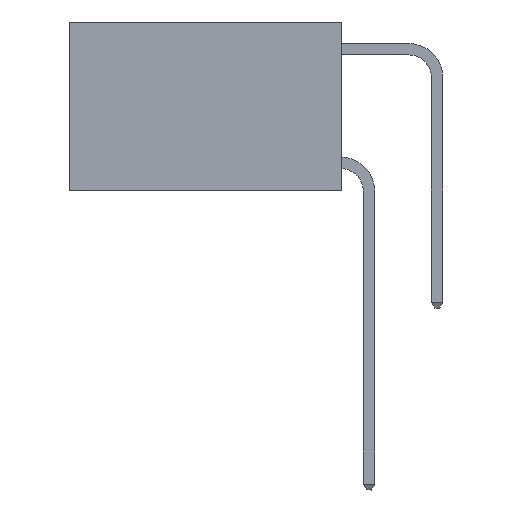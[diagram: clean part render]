
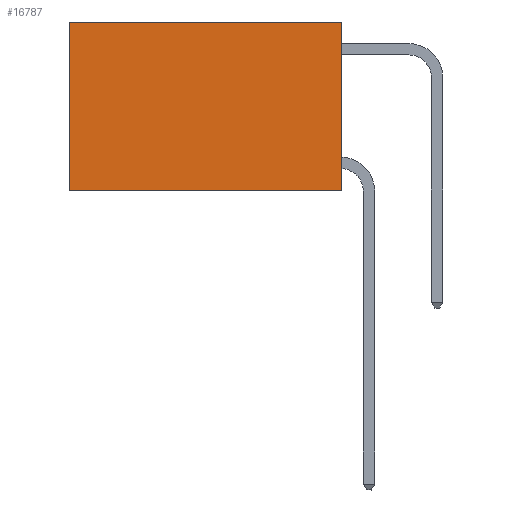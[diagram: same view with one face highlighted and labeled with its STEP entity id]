
A CAD part, left-side view. The second image highlights one B-rep face of the part: STEP entity #16787.
In plain terms, the highlighted planar face has unit normal (-1, 0, 0).
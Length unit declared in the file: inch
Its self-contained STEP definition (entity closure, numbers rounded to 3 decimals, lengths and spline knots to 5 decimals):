
#293 = CARTESIAN_POINT ( 'NONE',  ( 0.2625, 0., 0. ) ) ;
#444 = EDGE_CURVE ( 'NONE', #14229, #8735, #2460, .T. ) ;
#824 = CARTESIAN_POINT ( 'NONE',  ( 0.2625, 0., -0.37 ) ) ;
#1929 = CARTESIAN_POINT ( 'NONE',  ( 0.2625, 0., 0. ) ) ;
#2085 = EDGE_LOOP ( 'NONE', ( #18646, #18537, #19407, #20185 ) ) ;
#2142 = DIRECTION ( 'NONE',  ( 0., 0., -1. ) ) ;
#2460 = LINE ( 'NONE', #824, #11016 ) ;
#3606 = CARTESIAN_POINT ( 'NONE',  ( 0.2625, 0., 0. ) ) ;
#3950 = CARTESIAN_POINT ( 'NONE',  ( 0.2625, 0.6, 0. ) ) ;
#4005 = FACE_OUTER_BOUND ( 'NONE', #2085, .T. ) ;
#6518 = DIRECTION ( 'NONE',  ( 0., 0., -1. ) ) ;
#8426 = DIRECTION ( 'NONE',  ( 0., 1., 0. ) ) ;
#8735 = VERTEX_POINT ( 'NONE', #14678 ) ;
#8857 = EDGE_CURVE ( 'NONE', #22630, #14229, #11913, .T. ) ;
#9423 = DIRECTION ( 'NONE',  ( 0., 0., -1. ) ) ;
#9648 = VECTOR ( 'NONE', #6518, 39.37008 ) ;
#11016 = VECTOR ( 'NONE', #8426, 39.37008 ) ;
#11290 = AXIS2_PLACEMENT_3D ( 'NONE', #12656, #20361, #9423 ) ;
#11356 = VECTOR ( 'NONE', #2142, 39.37008 ) ;
#11913 = LINE ( 'NONE', #293, #11356 ) ;
#12656 = CARTESIAN_POINT ( 'NONE',  ( 0.2625, 0., 0. ) ) ;
#13918 = LINE ( 'NONE', #15612, #9648 ) ;
#14229 = VERTEX_POINT ( 'NONE', #16975 ) ;
#14528 = DIRECTION ( 'NONE',  ( 0., 1., 0. ) ) ;
#14678 = CARTESIAN_POINT ( 'NONE',  ( 0.2625, 0.6, -0.37 ) ) ;
#15612 = CARTESIAN_POINT ( 'NONE',  ( 0.2625, 0.6, 0. ) ) ;
#15707 = LINE ( 'NONE', #3606, #20563 ) ;
#16787 = ADVANCED_FACE ( 'NONE', ( #4005 ), #18216, .F. ) ;
#16975 = CARTESIAN_POINT ( 'NONE',  ( 0.2625, 0., -0.37 ) ) ;
#17814 = EDGE_CURVE ( 'NONE', #21885, #8735, #13918, .T. ) ;
#18216 = PLANE ( 'NONE',  #11290 ) ;
#18537 = ORIENTED_EDGE ( 'NONE', *, *, #444, .F. ) ;
#18646 = ORIENTED_EDGE ( 'NONE', *, *, #17814, .T. ) ;
#19407 = ORIENTED_EDGE ( 'NONE', *, *, #8857, .F. ) ;
#20185 = ORIENTED_EDGE ( 'NONE', *, *, #20463, .T. ) ;
#20361 = DIRECTION ( 'NONE',  ( 1., 0., 0. ) ) ;
#20463 = EDGE_CURVE ( 'NONE', #22630, #21885, #15707, .T. ) ;
#20563 = VECTOR ( 'NONE', #14528, 39.37008 ) ;
#21885 = VERTEX_POINT ( 'NONE', #3950 ) ;
#22630 = VERTEX_POINT ( 'NONE', #1929 ) ;
